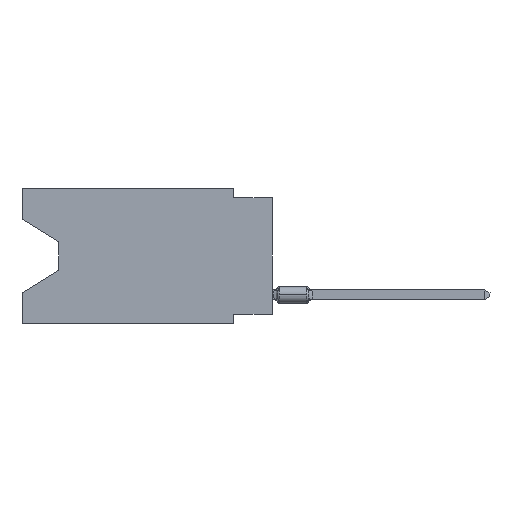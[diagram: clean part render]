
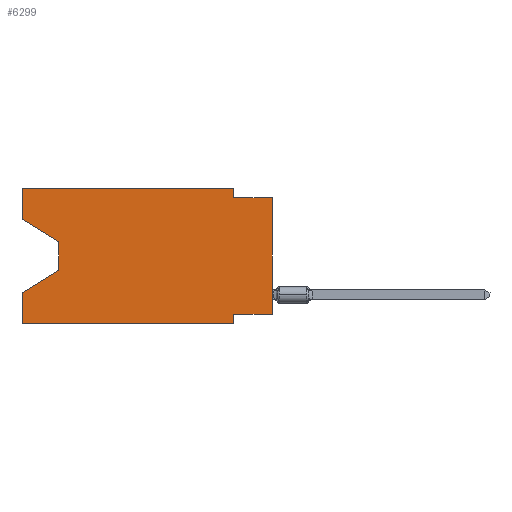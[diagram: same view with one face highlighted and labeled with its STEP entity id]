
A CAD part, left-side view. The second image highlights one B-rep face of the part: STEP entity #6299.
In plain terms, the highlighted planar face has unit normal (-1, 0, 0).
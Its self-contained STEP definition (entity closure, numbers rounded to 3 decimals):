
#163 = CARTESIAN_POINT ( 'NONE',  ( 0., 2.54, -0.635 ) ) ;
#180 = ORIENTED_EDGE ( 'NONE', *, *, #4828, .F. ) ;
#190 = DIRECTION ( 'NONE',  ( 0., -1., 0. ) ) ;
#262 = VECTOR ( 'NONE', #5826, 1000. ) ;
#525 = EDGE_CURVE ( 'NONE', #11328, #13139, #2413, .T. ) ;
#605 = CARTESIAN_POINT ( 'NONE',  ( 0., 13.97, -5.385 ) ) ;
#618 = ORIENTED_EDGE ( 'NONE', *, *, #15513, .F. ) ;
#640 = DIRECTION ( 'NONE',  ( 0., -1., 0. ) ) ;
#658 = CARTESIAN_POINT ( 'NONE',  ( 0., 16.383, 0. ) ) ;
#718 = CARTESIAN_POINT ( 'NONE',  ( 0., 16.383, 0. ) ) ;
#761 = CARTESIAN_POINT ( 'NONE',  ( 0., 0., 0. ) ) ;
#857 = ORIENTED_EDGE ( 'NONE', *, *, #11629, .T. ) ;
#1807 = VECTOR ( 'NONE', #8296, 1000. ) ;
#2283 = VERTEX_POINT ( 'NONE', #3962 ) ;
#2413 = LINE ( 'NONE', #7477, #2903 ) ;
#2457 = EDGE_CURVE ( 'NONE', #16204, #6901, #12073, .T. ) ;
#2534 = DIRECTION ( 'NONE',  ( 0., -1., 0. ) ) ;
#2744 = ORIENTED_EDGE ( 'NONE', *, *, #525, .T. ) ;
#2757 = CARTESIAN_POINT ( 'NONE',  ( 0., 16.383, -8.89 ) ) ;
#2903 = VECTOR ( 'NONE', #12532, 1000. ) ;
#3167 = VECTOR ( 'NONE', #14359, 1000. ) ;
#3171 = LINE ( 'NONE', #761, #262 ) ;
#3291 = EDGE_CURVE ( 'NONE', #3866, #14967, #5644, .T. ) ;
#3546 = CARTESIAN_POINT ( 'NONE',  ( 0., 16.383, -8.89 ) ) ;
#3866 = VERTEX_POINT ( 'NONE', #3546 ) ;
#3962 = CARTESIAN_POINT ( 'NONE',  ( 0., 16.383, 0. ) ) ;
#4402 = EDGE_CURVE ( 'NONE', #3866, #9664, #9140, .T. ) ;
#4631 = DIRECTION ( 'NONE',  ( 0., 0., 1. ) ) ;
#4828 = EDGE_CURVE ( 'NONE', #9592, #16204, #6719, .T. ) ;
#4877 = CARTESIAN_POINT ( 'NONE',  ( 0., 2.54, -8.89 ) ) ;
#4883 = CARTESIAN_POINT ( 'NONE',  ( 0., 16.383, 0. ) ) ;
#4953 = LINE ( 'NONE', #4883, #16124 ) ;
#4988 = VECTOR ( 'NONE', #4631, 1000. ) ;
#5367 = CARTESIAN_POINT ( 'NONE',  ( 0., 16.383, -2.038 ) ) ;
#5554 = VECTOR ( 'NONE', #10503, 1000. ) ;
#5644 = LINE ( 'NONE', #658, #1807 ) ;
#5663 = ORIENTED_EDGE ( 'NONE', *, *, #3291, .F. ) ;
#5826 = DIRECTION ( 'NONE',  ( 0., 0., 1. ) ) ;
#6256 = CARTESIAN_POINT ( 'NONE',  ( 0., 0., -0.635 ) ) ;
#6260 = LINE ( 'NONE', #6349, #11808 ) ;
#6299 = ADVANCED_FACE ( 'NONE', ( #12253 ), #10989, .F. ) ;
#6349 = CARTESIAN_POINT ( 'NONE',  ( 0., 13.97, -5.385 ) ) ;
#6393 = CARTESIAN_POINT ( 'NONE',  ( 0., 16.383, -6.852 ) ) ;
#6476 = EDGE_CURVE ( 'NONE', #2283, #9592, #4953, .T. ) ;
#6496 = VERTEX_POINT ( 'NONE', #5367 ) ;
#6719 = LINE ( 'NONE', #15393, #5554 ) ;
#6901 = VERTEX_POINT ( 'NONE', #6256 ) ;
#6956 = DIRECTION ( 'NONE',  ( 0., 0., -1. ) ) ;
#7069 = CARTESIAN_POINT ( 'NONE',  ( 0., 2.54, -8.89 ) ) ;
#7140 = AXIS2_PLACEMENT_3D ( 'NONE', #718, #10833, #6956 ) ;
#7173 = ORIENTED_EDGE ( 'NONE', *, *, #13510, .F. ) ;
#7323 = CARTESIAN_POINT ( 'NONE',  ( 0., 16.383, -2.038 ) ) ;
#7477 = CARTESIAN_POINT ( 'NONE',  ( 0., 13.97, -3.505 ) ) ;
#7977 = CARTESIAN_POINT ( 'NONE',  ( 0., 16.383, 0. ) ) ;
#8083 = EDGE_CURVE ( 'NONE', #13139, #14967, #6260, .T. ) ;
#8296 = DIRECTION ( 'NONE',  ( 0., 0., 1. ) ) ;
#8432 = CARTESIAN_POINT ( 'NONE',  ( 0., 0., -8.255 ) ) ;
#8583 = DIRECTION ( 'NONE',  ( 0., -0.855, -0.519 ) ) ;
#9140 = LINE ( 'NONE', #2757, #11353 ) ;
#9261 = ORIENTED_EDGE ( 'NONE', *, *, #11441, .F. ) ;
#9322 = ORIENTED_EDGE ( 'NONE', *, *, #6476, .F. ) ;
#9592 = VERTEX_POINT ( 'NONE', #9843 ) ;
#9664 = VERTEX_POINT ( 'NONE', #4877 ) ;
#9843 = CARTESIAN_POINT ( 'NONE',  ( 0., 2.54, 0. ) ) ;
#10139 = EDGE_CURVE ( 'NONE', #6496, #11328, #14866, .T. ) ;
#10454 = ORIENTED_EDGE ( 'NONE', *, *, #2457, .F. ) ;
#10503 = DIRECTION ( 'NONE',  ( 0., 0., -1. ) ) ;
#10833 = DIRECTION ( 'NONE',  ( 1., 0., 0. ) ) ;
#10911 = CARTESIAN_POINT ( 'NONE',  ( 0., 0., -0.635 ) ) ;
#10989 = PLANE ( 'NONE',  #7140 ) ;
#11192 = ORIENTED_EDGE ( 'NONE', *, *, #10139, .T. ) ;
#11328 = VERTEX_POINT ( 'NONE', #11463 ) ;
#11353 = VECTOR ( 'NONE', #190, 1000. ) ;
#11441 = EDGE_CURVE ( 'NONE', #12466, #11726, #14114, .T. ) ;
#11463 = CARTESIAN_POINT ( 'NONE',  ( 0., 13.97, -3.505 ) ) ;
#11629 = EDGE_CURVE ( 'NONE', #12466, #6901, #3171, .T. ) ;
#11726 = VERTEX_POINT ( 'NONE', #14998 ) ;
#11808 = VECTOR ( 'NONE', #16350, 1000. ) ;
#12073 = LINE ( 'NONE', #10911, #14600 ) ;
#12120 = DIRECTION ( 'NONE',  ( 0., 0., -1. ) ) ;
#12253 = FACE_OUTER_BOUND ( 'NONE', #14717, .T. ) ;
#12466 = VERTEX_POINT ( 'NONE', #8432 ) ;
#12532 = DIRECTION ( 'NONE',  ( 0., 0., -1. ) ) ;
#13118 = CARTESIAN_POINT ( 'NONE',  ( 0., 0., -8.255 ) ) ;
#13139 = VERTEX_POINT ( 'NONE', #605 ) ;
#13186 = VECTOR ( 'NONE', #8583, 1000. ) ;
#13239 = ORIENTED_EDGE ( 'NONE', *, *, #4402, .T. ) ;
#13494 = LINE ( 'NONE', #7977, #4988 ) ;
#13510 = EDGE_CURVE ( 'NONE', #6496, #2283, #13494, .T. ) ;
#14047 = VECTOR ( 'NONE', #12120, 1000. ) ;
#14114 = LINE ( 'NONE', #13118, #3167 ) ;
#14359 = DIRECTION ( 'NONE',  ( 0., 1., 0. ) ) ;
#14437 = LINE ( 'NONE', #7069, #14047 ) ;
#14600 = VECTOR ( 'NONE', #640, 1000. ) ;
#14717 = EDGE_LOOP ( 'NONE', ( #11192, #2744, #15934, #5663, #13239, #618, #9261, #857, #10454, #180, #9322, #7173 ) ) ;
#14866 = LINE ( 'NONE', #7323, #13186 ) ;
#14967 = VERTEX_POINT ( 'NONE', #6393 ) ;
#14998 = CARTESIAN_POINT ( 'NONE',  ( 0., 2.54, -8.255 ) ) ;
#15393 = CARTESIAN_POINT ( 'NONE',  ( 0., 2.54, 0. ) ) ;
#15513 = EDGE_CURVE ( 'NONE', #11726, #9664, #14437, .T. ) ;
#15934 = ORIENTED_EDGE ( 'NONE', *, *, #8083, .T. ) ;
#16124 = VECTOR ( 'NONE', #2534, 1000. ) ;
#16204 = VERTEX_POINT ( 'NONE', #163 ) ;
#16350 = DIRECTION ( 'NONE',  ( 0., 0.855, -0.519 ) ) ;
